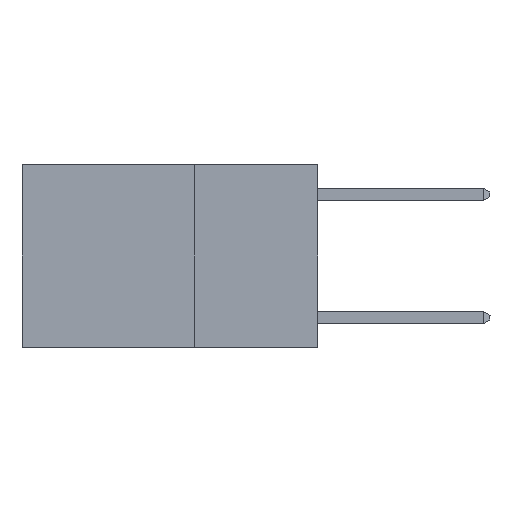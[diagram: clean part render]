
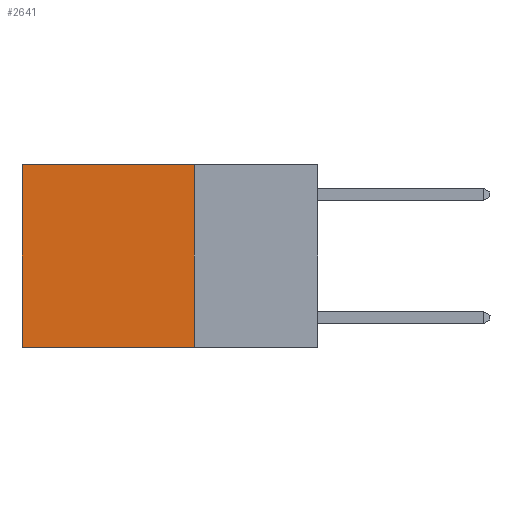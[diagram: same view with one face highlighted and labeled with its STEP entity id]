
A CAD part, left-side view. The second image highlights one B-rep face of the part: STEP entity #2641.
In plain terms, the highlighted planar face has unit normal (-1, 0, 0).
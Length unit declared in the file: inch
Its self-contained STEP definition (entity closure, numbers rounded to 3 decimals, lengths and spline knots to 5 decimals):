
#192 = ORIENTED_EDGE ( 'NONE', *, *, #2969, .T. ) ;
#1250 = CARTESIAN_POINT ( 'NONE',  ( 0.2625, 0.25, -0.37 ) ) ;
#1431 = VERTEX_POINT ( 'NONE', #2409 ) ;
#1558 = PLANE ( 'NONE',  #3863 ) ;
#1673 = DIRECTION ( 'NONE',  ( 0., 0., -1. ) ) ;
#2049 = DIRECTION ( 'NONE',  ( 0., 0., -1. ) ) ;
#2308 = CARTESIAN_POINT ( 'NONE',  ( 0.2625, 0.6, 0. ) ) ;
#2409 = CARTESIAN_POINT ( 'NONE',  ( 0.2625, 0.25, 0. ) ) ;
#2641 = ADVANCED_FACE ( 'NONE', ( #14212 ), #1558, .F. ) ;
#2866 = EDGE_CURVE ( 'NONE', #1431, #3439, #16138, .T. ) ;
#2969 = EDGE_CURVE ( 'NONE', #1431, #10311, #12482, .T. ) ;
#3439 = VERTEX_POINT ( 'NONE', #15062 ) ;
#3863 = AXIS2_PLACEMENT_3D ( 'NONE', #15263, #4371, #1673 ) ;
#4157 = EDGE_LOOP ( 'NONE', ( #6555, #16599, #16986, #192 ) ) ;
#4371 = DIRECTION ( 'NONE',  ( 1., 0., 0. ) ) ;
#4753 = VERTEX_POINT ( 'NONE', #6180 ) ;
#6180 = CARTESIAN_POINT ( 'NONE',  ( 0.2625, 0.6, -0.37 ) ) ;
#6555 = ORIENTED_EDGE ( 'NONE', *, *, #14516, .T. ) ;
#6636 = DIRECTION ( 'NONE',  ( 0., 1., 0. ) ) ;
#6641 = VECTOR ( 'NONE', #2049, 39.37008 ) ;
#7134 = VECTOR ( 'NONE', #8239, 39.37008 ) ;
#8239 = DIRECTION ( 'NONE',  ( 0., 1., 0. ) ) ;
#8319 = EDGE_CURVE ( 'NONE', #3439, #4753, #9013, .T. ) ;
#8813 = LINE ( 'NONE', #2308, #6641 ) ;
#8957 = CARTESIAN_POINT ( 'NONE',  ( 0.2625, 0.25, 0. ) ) ;
#9013 = LINE ( 'NONE', #1250, #10951 ) ;
#10311 = VERTEX_POINT ( 'NONE', #13472 ) ;
#10408 = DIRECTION ( 'NONE',  ( 0., 0., -1. ) ) ;
#10761 = VECTOR ( 'NONE', #10408, 39.37008 ) ;
#10951 = VECTOR ( 'NONE', #6636, 39.37008 ) ;
#12482 = LINE ( 'NONE', #16463, #7134 ) ;
#13472 = CARTESIAN_POINT ( 'NONE',  ( 0.2625, 0.6, 0. ) ) ;
#14212 = FACE_OUTER_BOUND ( 'NONE', #4157, .T. ) ;
#14516 = EDGE_CURVE ( 'NONE', #10311, #4753, #8813, .T. ) ;
#15062 = CARTESIAN_POINT ( 'NONE',  ( 0.2625, 0.25, -0.37 ) ) ;
#15263 = CARTESIAN_POINT ( 'NONE',  ( 0.2625, 0.25, 0. ) ) ;
#16138 = LINE ( 'NONE', #8957, #10761 ) ;
#16463 = CARTESIAN_POINT ( 'NONE',  ( 0.2625, 0.25, 0. ) ) ;
#16599 = ORIENTED_EDGE ( 'NONE', *, *, #8319, .F. ) ;
#16986 = ORIENTED_EDGE ( 'NONE', *, *, #2866, .F. ) ;
